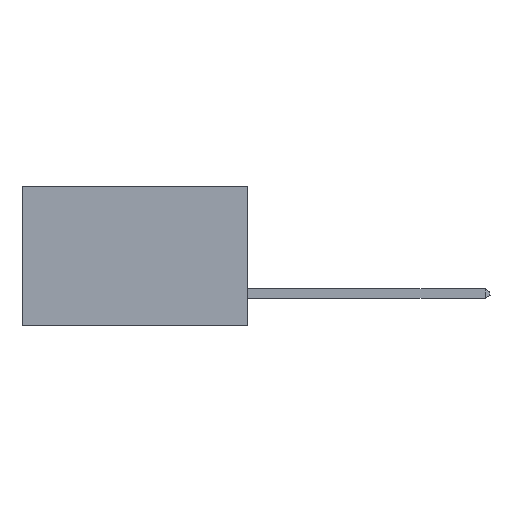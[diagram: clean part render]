
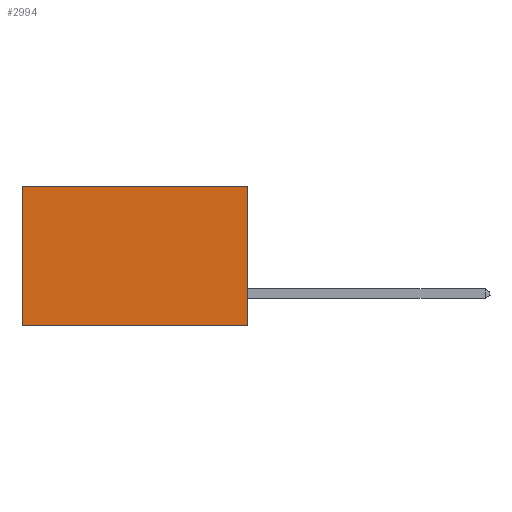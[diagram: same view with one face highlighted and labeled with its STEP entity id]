
A CAD part, left-side view. The second image highlights one B-rep face of the part: STEP entity #2994.
In plain terms, the highlighted planar face has unit normal (-1, 0, 0).
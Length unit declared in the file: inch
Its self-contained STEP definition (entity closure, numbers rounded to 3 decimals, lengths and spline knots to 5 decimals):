
#23 = FACE_OUTER_BOUND ( 'NONE', #8617, .T. ) ;
#24 = EDGE_CURVE ( 'NONE', #2390, #3835, #6637, .T. ) ;
#348 = VECTOR ( 'NONE', #10676, 39.37008 ) ;
#400 = DIRECTION ( 'NONE',  ( 0., 1., 0. ) ) ;
#607 = DIRECTION ( 'NONE',  ( 0., 0., -1. ) ) ;
#942 = CARTESIAN_POINT ( 'NONE',  ( 0.298, 0.6, 0. ) ) ;
#988 = VECTOR ( 'NONE', #400, 39.37008 ) ;
#1049 = ORIENTED_EDGE ( 'NONE', *, *, #24, .F. ) ;
#1550 = EDGE_CURVE ( 'NONE', #5935, #2390, #2109, .T. ) ;
#1655 = ORIENTED_EDGE ( 'NONE', *, *, #9531, .T. ) ;
#2109 = LINE ( 'NONE', #10635, #348 ) ;
#2390 = VERTEX_POINT ( 'NONE', #8306 ) ;
#2411 = PLANE ( 'NONE',  #5371 ) ;
#2697 = VECTOR ( 'NONE', #8286, 39.37008 ) ;
#2835 = LINE ( 'NONE', #5591, #2697 ) ;
#2981 = CARTESIAN_POINT ( 'NONE',  ( 0.298, 0.6, -0.37 ) ) ;
#2994 = ADVANCED_FACE ( 'NONE', ( #23 ), #2411, .F. ) ;
#3440 = ORIENTED_EDGE ( 'NONE', *, *, #4352, .T. ) ;
#3537 = VECTOR ( 'NONE', #5448, 39.37008 ) ;
#3835 = VERTEX_POINT ( 'NONE', #2981 ) ;
#4098 = VERTEX_POINT ( 'NONE', #8167 ) ;
#4112 = ORIENTED_EDGE ( 'NONE', *, *, #1550, .F. ) ;
#4352 = EDGE_CURVE ( 'NONE', #4098, #3835, #4954, .T. ) ;
#4954 = LINE ( 'NONE', #942, #3537 ) ;
#5371 = AXIS2_PLACEMENT_3D ( 'NONE', #9465, #9661, #607 ) ;
#5396 = CARTESIAN_POINT ( 'NONE',  ( 0.298, 0., 0. ) ) ;
#5448 = DIRECTION ( 'NONE',  ( 0., 0., -1. ) ) ;
#5591 = CARTESIAN_POINT ( 'NONE',  ( 0.298, 0., 0. ) ) ;
#5662 = CARTESIAN_POINT ( 'NONE',  ( 0.298, 0., -0.37 ) ) ;
#5935 = VERTEX_POINT ( 'NONE', #5396 ) ;
#6637 = LINE ( 'NONE', #5662, #988 ) ;
#8167 = CARTESIAN_POINT ( 'NONE',  ( 0.298, 0.6, 0. ) ) ;
#8286 = DIRECTION ( 'NONE',  ( 0., 1., 0. ) ) ;
#8306 = CARTESIAN_POINT ( 'NONE',  ( 0.298, 0., -0.37 ) ) ;
#8617 = EDGE_LOOP ( 'NONE', ( #3440, #1049, #4112, #1655 ) ) ;
#9465 = CARTESIAN_POINT ( 'NONE',  ( 0.298, 0., 0. ) ) ;
#9531 = EDGE_CURVE ( 'NONE', #5935, #4098, #2835, .T. ) ;
#9661 = DIRECTION ( 'NONE',  ( 1., 0., 0. ) ) ;
#10635 = CARTESIAN_POINT ( 'NONE',  ( 0.298, 0., 0. ) ) ;
#10676 = DIRECTION ( 'NONE',  ( 0., 0., -1. ) ) ;
